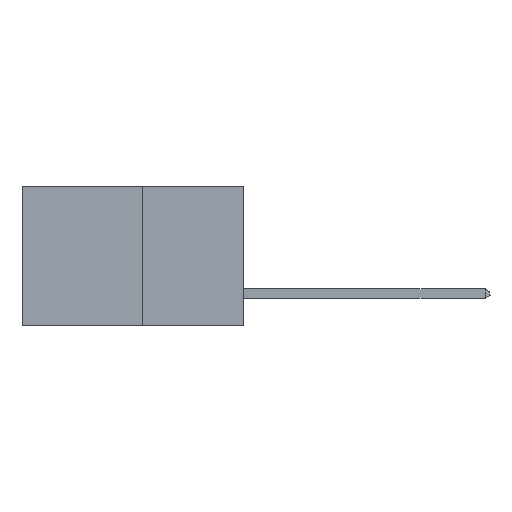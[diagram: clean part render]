
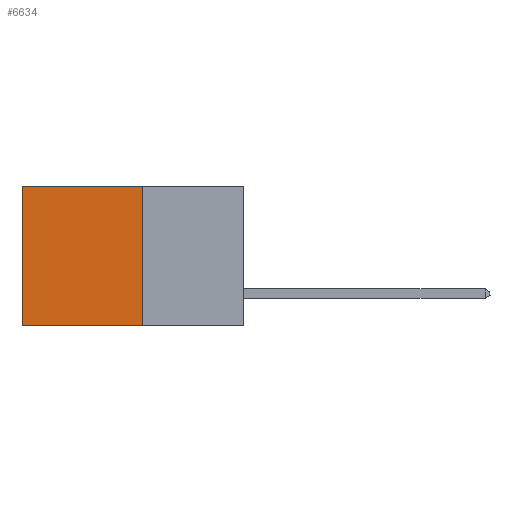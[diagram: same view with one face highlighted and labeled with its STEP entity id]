
A CAD part, left-side view. The second image highlights one B-rep face of the part: STEP entity #6634.
In plain terms, the highlighted planar face has unit normal (-1, 0, 0).
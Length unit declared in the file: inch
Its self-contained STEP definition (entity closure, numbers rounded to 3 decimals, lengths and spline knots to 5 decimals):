
#372 = ORIENTED_EDGE ( 'NONE', *, *, #1458, .F. ) ;
#486 = EDGE_CURVE ( 'NONE', #4089, #5663, #6783, .T. ) ;
#630 = CARTESIAN_POINT ( 'NONE',  ( 0.277, 0.27, 0. ) ) ;
#1458 = EDGE_CURVE ( 'NONE', #8729, #4089, #2938, .T. ) ;
#1977 = CARTESIAN_POINT ( 'NONE',  ( 0.277, 0.59, 0. ) ) ;
#2938 = LINE ( 'NONE', #12001, #3305 ) ;
#3197 = ORIENTED_EDGE ( 'NONE', *, *, #486, .F. ) ;
#3297 = PLANE ( 'NONE',  #10879 ) ;
#3305 = VECTOR ( 'NONE', #11806, 39.37008 ) ;
#3570 = ORIENTED_EDGE ( 'NONE', *, *, #3889, .T. ) ;
#3889 = EDGE_CURVE ( 'NONE', #8729, #5742, #9051, .T. ) ;
#4089 = VERTEX_POINT ( 'NONE', #12542 ) ;
#4633 = CARTESIAN_POINT ( 'NONE',  ( 0.277, 0.59, -0.37 ) ) ;
#5663 = VERTEX_POINT ( 'NONE', #6364 ) ;
#5742 = VERTEX_POINT ( 'NONE', #1977 ) ;
#5818 = DIRECTION ( 'NONE',  ( 0., 1., 0. ) ) ;
#5891 = FACE_OUTER_BOUND ( 'NONE', #12331, .T. ) ;
#6216 = VECTOR ( 'NONE', #6678, 39.37008 ) ;
#6364 = CARTESIAN_POINT ( 'NONE',  ( 0.277, 0.59, -0.37 ) ) ;
#6458 = VECTOR ( 'NONE', #13559, 39.37008 ) ;
#6631 = DIRECTION ( 'NONE',  ( 1., 0., 0. ) ) ;
#6634 = ADVANCED_FACE ( 'NONE', ( #5891 ), #3297, .F. ) ;
#6678 = DIRECTION ( 'NONE',  ( 0., 0., -1. ) ) ;
#6783 = LINE ( 'NONE', #11503, #6458 ) ;
#8729 = VERTEX_POINT ( 'NONE', #630 ) ;
#9051 = LINE ( 'NONE', #12053, #11815 ) ;
#10776 = EDGE_CURVE ( 'NONE', #5742, #5663, #11757, .T. ) ;
#10879 = AXIS2_PLACEMENT_3D ( 'NONE', #12848, #6631, #13876 ) ;
#11372 = ORIENTED_EDGE ( 'NONE', *, *, #10776, .T. ) ;
#11503 = CARTESIAN_POINT ( 'NONE',  ( 0.277, 0.27, -0.37 ) ) ;
#11757 = LINE ( 'NONE', #4633, #6216 ) ;
#11806 = DIRECTION ( 'NONE',  ( 0., 0., -1. ) ) ;
#11815 = VECTOR ( 'NONE', #5818, 39.37008 ) ;
#12001 = CARTESIAN_POINT ( 'NONE',  ( 0.277, 0.27, -0.37 ) ) ;
#12053 = CARTESIAN_POINT ( 'NONE',  ( 0.277, 0.27, 0. ) ) ;
#12331 = EDGE_LOOP ( 'NONE', ( #11372, #3197, #372, #3570 ) ) ;
#12542 = CARTESIAN_POINT ( 'NONE',  ( 0.277, 0.27, -0.37 ) ) ;
#12848 = CARTESIAN_POINT ( 'NONE',  ( 0.277, 0.27, -0.37 ) ) ;
#13559 = DIRECTION ( 'NONE',  ( 0., 1., 0. ) ) ;
#13876 = DIRECTION ( 'NONE',  ( 0., 0., -1. ) ) ;
